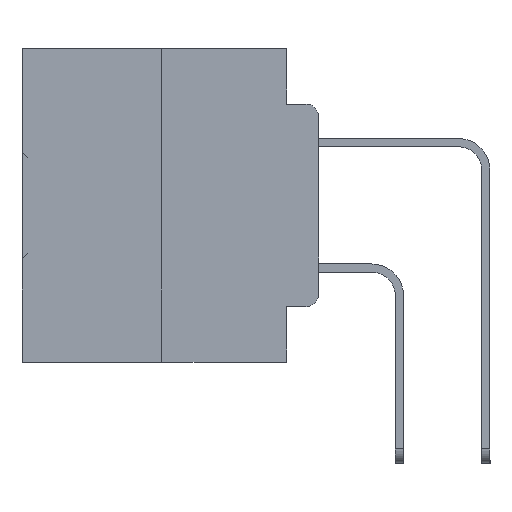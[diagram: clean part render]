
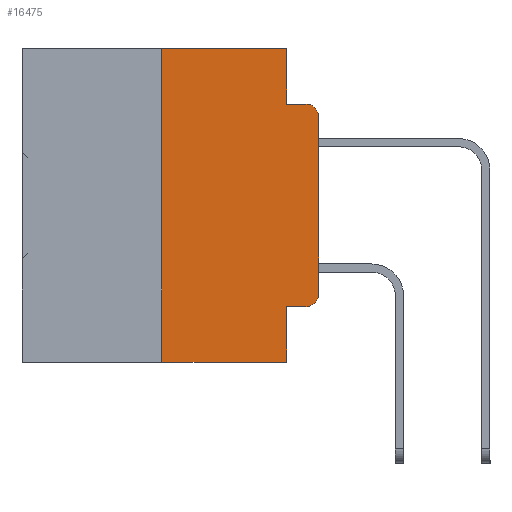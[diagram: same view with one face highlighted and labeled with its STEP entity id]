
A CAD part, left-side view. The second image highlights one B-rep face of the part: STEP entity #16475.
In plain terms, the highlighted planar face has unit normal (-1, 0, 0).
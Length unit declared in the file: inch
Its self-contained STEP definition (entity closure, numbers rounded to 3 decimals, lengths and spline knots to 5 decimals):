
#240 = VECTOR ( 'NONE', #12075, 39.37008 ) ;
#862 = EDGE_CURVE ( 'NONE', #20683, #35349, #7595, .T. ) ;
#1974 = LINE ( 'NONE', #21506, #8113 ) ;
#3024 = CARTESIAN_POINT ( 'NONE',  ( 0., 0.051, -0.4115 ) ) ;
#3640 = CARTESIAN_POINT ( 'NONE',  ( 0., 0.02, -0.3915 ) ) ;
#3805 = ORIENTED_EDGE ( 'NONE', *, *, #38175, .F. ) ;
#4683 = AXIS2_PLACEMENT_3D ( 'NONE', #28562, #10609, #31534 ) ;
#4986 = VECTOR ( 'NONE', #30283, 39.37008 ) ;
#5574 = VECTOR ( 'NONE', #13858, 39.37008 ) ;
#6030 = VERTEX_POINT ( 'NONE', #14600 ) ;
#6538 = LINE ( 'NONE', #28764, #5574 ) ;
#6686 = DIRECTION ( 'NONE',  ( 0., 0., -1. ) ) ;
#7396 = DIRECTION ( 'NONE',  ( 1., 0., 0. ) ) ;
#7595 = LINE ( 'NONE', #13678, #15592 ) ;
#7642 = CARTESIAN_POINT ( 'NONE',  ( 0., 0.25, -0.5 ) ) ;
#8062 = ORIENTED_EDGE ( 'NONE', *, *, #36194, .F. ) ;
#8113 = VECTOR ( 'NONE', #9594, 39.37008 ) ;
#9009 = DIRECTION ( 'NONE',  ( 0., -1., 0. ) ) ;
#9054 = CARTESIAN_POINT ( 'NONE',  ( 0., 0., 0. ) ) ;
#9594 = DIRECTION ( 'NONE',  ( 0., -1., 0. ) ) ;
#9772 = CARTESIAN_POINT ( 'NONE',  ( 0., 0.02, -0.4115 ) ) ;
#9911 = ORIENTED_EDGE ( 'NONE', *, *, #30121, .F. ) ;
#10609 = DIRECTION ( 'NONE',  ( -1., 0., 0. ) ) ;
#11520 = VERTEX_POINT ( 'NONE', #33797 ) ;
#11974 = VERTEX_POINT ( 'NONE', #18210 ) ;
#12075 = DIRECTION ( 'NONE',  ( 0., 0., 1. ) ) ;
#13112 = VERTEX_POINT ( 'NONE', #26654 ) ;
#13475 = VECTOR ( 'NONE', #21179, 39.37008 ) ;
#13678 = CARTESIAN_POINT ( 'NONE',  ( 0., 0.473, -0.5 ) ) ;
#13858 = DIRECTION ( 'NONE',  ( 0., 0., -1. ) ) ;
#14491 = VERTEX_POINT ( 'NONE', #9772 ) ;
#14600 = CARTESIAN_POINT ( 'NONE',  ( 0., 0., -0.3915 ) ) ;
#15583 = CARTESIAN_POINT ( 'NONE',  ( 0., 0.473, 0. ) ) ;
#15592 = VECTOR ( 'NONE', #9009, 39.37008 ) ;
#15985 = CIRCLE ( 'NONE', #4683, 0.02 ) ;
#16282 = FACE_OUTER_BOUND ( 'NONE', #29272, .T. ) ;
#16475 = ADVANCED_FACE ( 'NONE', ( #16282 ), #34348, .F. ) ;
#16522 = AXIS2_PLACEMENT_3D ( 'NONE', #37176, #7396, #37306 ) ;
#17462 = EDGE_CURVE ( 'NONE', #11974, #11520, #36787, .T. ) ;
#17858 = VECTOR ( 'NONE', #23652, 39.37008 ) ;
#18198 = EDGE_CURVE ( 'NONE', #14491, #6030, #18541, .T. ) ;
#18210 = CARTESIAN_POINT ( 'NONE',  ( 0., 0.051, 0. ) ) ;
#18541 = CIRCLE ( 'NONE', #29354, 0.02 ) ;
#19471 = EDGE_CURVE ( 'NONE', #11520, #13112, #1974, .T. ) ;
#20495 = VERTEX_POINT ( 'NONE', #27589 ) ;
#20683 = VERTEX_POINT ( 'NONE', #7642 ) ;
#20701 = LINE ( 'NONE', #15583, #27339 ) ;
#21179 = DIRECTION ( 'NONE',  ( 0., 0., 1. ) ) ;
#21506 = CARTESIAN_POINT ( 'NONE',  ( 0., 0.051, -0.0885 ) ) ;
#22209 = EDGE_CURVE ( 'NONE', #36430, #14491, #26761, .T. ) ;
#23652 = DIRECTION ( 'NONE',  ( 0., -1., 0. ) ) ;
#23978 = ORIENTED_EDGE ( 'NONE', *, *, #17462, .F. ) ;
#24297 = CARTESIAN_POINT ( 'NONE',  ( 0., 0.051, 0. ) ) ;
#24440 = VERTEX_POINT ( 'NONE', #36551 ) ;
#24626 = DIRECTION ( 'NONE',  ( -1., 0., 0. ) ) ;
#24882 = ORIENTED_EDGE ( 'NONE', *, *, #35458, .T. ) ;
#25891 = ORIENTED_EDGE ( 'NONE', *, *, #22209, .T. ) ;
#26654 = CARTESIAN_POINT ( 'NONE',  ( 0., 0.02, -0.0885 ) ) ;
#26761 = LINE ( 'NONE', #38472, #17858 ) ;
#27339 = VECTOR ( 'NONE', #30483, 39.37008 ) ;
#27589 = CARTESIAN_POINT ( 'NONE',  ( 0., 0., -0.1085 ) ) ;
#27921 = CARTESIAN_POINT ( 'NONE',  ( 0., 0.051, -0.5 ) ) ;
#28562 = CARTESIAN_POINT ( 'NONE',  ( 0., 0.02, -0.1085 ) ) ;
#28764 = CARTESIAN_POINT ( 'NONE',  ( 0., 0.051, 0. ) ) ;
#29272 = EDGE_LOOP ( 'NONE', ( #36964, #24882, #37443, #23978, #9911, #3805, #34267, #8062, #25891, #32768 ) ) ;
#29354 = AXIS2_PLACEMENT_3D ( 'NONE', #3640, #24626, #6686 ) ;
#29367 = LINE ( 'NONE', #33199, #13475 ) ;
#30121 = EDGE_CURVE ( 'NONE', #24440, #11974, #20701, .T. ) ;
#30283 = DIRECTION ( 'NONE',  ( 0., 0., -1. ) ) ;
#30483 = DIRECTION ( 'NONE',  ( 0., -1., 0. ) ) ;
#31534 = DIRECTION ( 'NONE',  ( 0., 0., -1. ) ) ;
#32768 = ORIENTED_EDGE ( 'NONE', *, *, #18198, .T. ) ;
#33199 = CARTESIAN_POINT ( 'NONE',  ( 0., 0.25, 0. ) ) ;
#33797 = CARTESIAN_POINT ( 'NONE',  ( 0., 0.051, -0.0885 ) ) ;
#34267 = ORIENTED_EDGE ( 'NONE', *, *, #862, .T. ) ;
#34348 = PLANE ( 'NONE',  #16522 ) ;
#35349 = VERTEX_POINT ( 'NONE', #27921 ) ;
#35458 = EDGE_CURVE ( 'NONE', #20495, #13112, #15985, .T. ) ;
#36194 = EDGE_CURVE ( 'NONE', #36430, #35349, #6538, .T. ) ;
#36430 = VERTEX_POINT ( 'NONE', #3024 ) ;
#36551 = CARTESIAN_POINT ( 'NONE',  ( 0., 0.25, 0. ) ) ;
#36787 = LINE ( 'NONE', #24297, #4986 ) ;
#36964 = ORIENTED_EDGE ( 'NONE', *, *, #37441, .T. ) ;
#37176 = CARTESIAN_POINT ( 'NONE',  ( 0., 0.473, 0. ) ) ;
#37306 = DIRECTION ( 'NONE',  ( 0., 0., -1. ) ) ;
#37441 = EDGE_CURVE ( 'NONE', #6030, #20495, #38186, .T. ) ;
#37443 = ORIENTED_EDGE ( 'NONE', *, *, #19471, .F. ) ;
#38175 = EDGE_CURVE ( 'NONE', #20683, #24440, #29367, .T. ) ;
#38186 = LINE ( 'NONE', #9054, #240 ) ;
#38472 = CARTESIAN_POINT ( 'NONE',  ( 0., 0.051, -0.4115 ) ) ;
